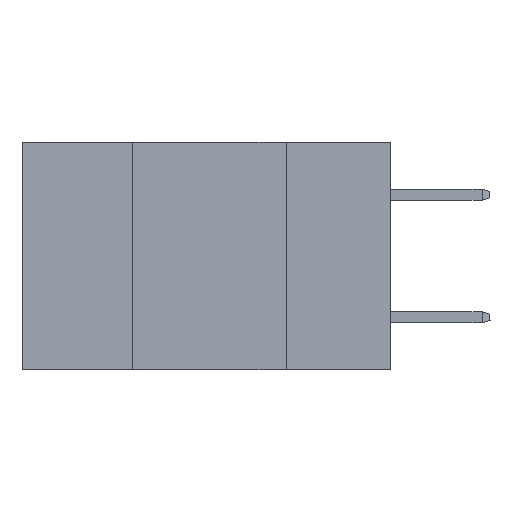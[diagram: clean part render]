
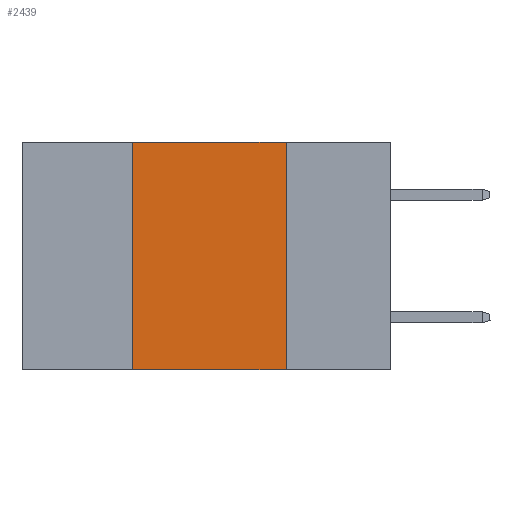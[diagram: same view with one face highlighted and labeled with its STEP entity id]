
A CAD part, left-side view. The second image highlights one B-rep face of the part: STEP entity #2439.
In plain terms, the highlighted planar face has unit normal (-1, 0, 0).
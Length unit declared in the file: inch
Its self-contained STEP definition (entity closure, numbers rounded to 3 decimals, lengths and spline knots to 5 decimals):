
#37 = LINE ( 'NONE', #22326, #1203 ) ;
#435 = VERTEX_POINT ( 'NONE', #3478 ) ;
#1148 = CARTESIAN_POINT ( 'NONE',  ( 0., 0.17, 0. ) ) ;
#1153 = DIRECTION ( 'NONE',  ( 0., -1., 0. ) ) ;
#1203 = VECTOR ( 'NONE', #22403, 39.37008 ) ;
#1865 = EDGE_CURVE ( 'NONE', #9743, #17935, #13185, .T. ) ;
#1921 = VECTOR ( 'NONE', #4582, 39.37008 ) ;
#2439 = ADVANCED_FACE ( 'NONE', ( #4415 ), #18149, .F. ) ;
#2470 = CARTESIAN_POINT ( 'NONE',  ( 0., 0.6, 0. ) ) ;
#2908 = CARTESIAN_POINT ( 'NONE',  ( 0., 0.6, -0.37 ) ) ;
#3478 = CARTESIAN_POINT ( 'NONE',  ( 0., 0.17, -0.37 ) ) ;
#4415 = FACE_OUTER_BOUND ( 'NONE', #13350, .T. ) ;
#4487 = LINE ( 'NONE', #2908, #1921 ) ;
#4582 = DIRECTION ( 'NONE',  ( 0., -1., 0. ) ) ;
#4739 = VERTEX_POINT ( 'NONE', #4810 ) ;
#4810 = CARTESIAN_POINT ( 'NONE',  ( 0., 0.42, -0.37 ) ) ;
#5348 = VECTOR ( 'NONE', #1153, 39.37008 ) ;
#7145 = EDGE_CURVE ( 'NONE', #4739, #435, #4487, .T. ) ;
#7934 = DIRECTION ( 'NONE',  ( 0., 0., -1. ) ) ;
#9743 = VERTEX_POINT ( 'NONE', #13802 ) ;
#11715 = CARTESIAN_POINT ( 'NONE',  ( 0., 0.17, 0. ) ) ;
#11914 = EDGE_CURVE ( 'NONE', #17935, #435, #12792, .T. ) ;
#12725 = DIRECTION ( 'NONE',  ( 1., 0., 0. ) ) ;
#12792 = LINE ( 'NONE', #1148, #14547 ) ;
#13185 = LINE ( 'NONE', #2470, #5348 ) ;
#13350 = EDGE_LOOP ( 'NONE', ( #18903, #20719, #22565, #16523 ) ) ;
#13661 = EDGE_CURVE ( 'NONE', #4739, #9743, #37, .T. ) ;
#13802 = CARTESIAN_POINT ( 'NONE',  ( 0., 0.42, 0. ) ) ;
#14547 = VECTOR ( 'NONE', #7934, 39.37008 ) ;
#15966 = AXIS2_PLACEMENT_3D ( 'NONE', #21992, #12725, #20010 ) ;
#16523 = ORIENTED_EDGE ( 'NONE', *, *, #7145, .T. ) ;
#17935 = VERTEX_POINT ( 'NONE', #11715 ) ;
#18149 = PLANE ( 'NONE',  #15966 ) ;
#18903 = ORIENTED_EDGE ( 'NONE', *, *, #11914, .F. ) ;
#20010 = DIRECTION ( 'NONE',  ( 0., 0., -1. ) ) ;
#20719 = ORIENTED_EDGE ( 'NONE', *, *, #1865, .F. ) ;
#21992 = CARTESIAN_POINT ( 'NONE',  ( 0., 0.6, 0. ) ) ;
#22326 = CARTESIAN_POINT ( 'NONE',  ( 0., 0.42, 0. ) ) ;
#22403 = DIRECTION ( 'NONE',  ( 0., 0., 1. ) ) ;
#22565 = ORIENTED_EDGE ( 'NONE', *, *, #13661, .F. ) ;
